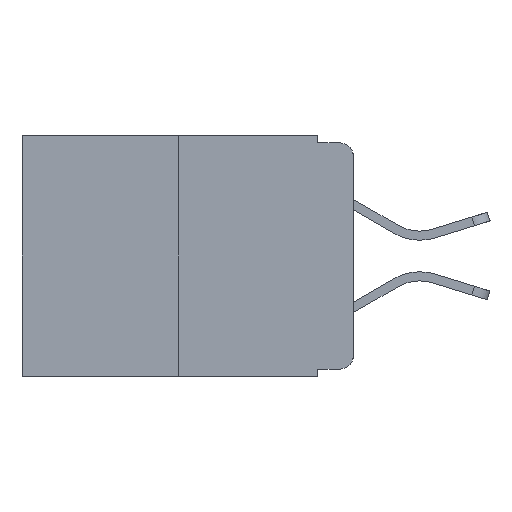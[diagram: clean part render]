
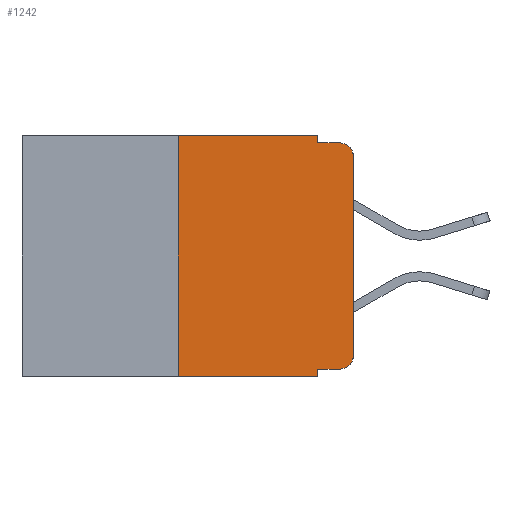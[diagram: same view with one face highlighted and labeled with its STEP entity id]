
A CAD part, left-side view. The second image highlights one B-rep face of the part: STEP entity #1242.
In plain terms, the highlighted planar face has unit normal (-1, 0, 0).
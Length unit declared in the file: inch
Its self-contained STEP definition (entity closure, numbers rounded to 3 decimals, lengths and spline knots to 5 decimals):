
#228 = DIRECTION ( 'NONE',  ( -1., 0., 0. ) ) ;
#306 = CARTESIAN_POINT ( 'NONE',  ( 0., 0.02, -0.333 ) ) ;
#309 = ORIENTED_EDGE ( 'NONE', *, *, #1476, .F. ) ;
#328 = DIRECTION ( 'NONE',  ( 0., 0., -1. ) ) ;
#923 = ORIENTED_EDGE ( 'NONE', *, *, #10424, .F. ) ;
#1242 = ADVANCED_FACE ( 'NONE', ( #10671 ), #13701, .F. ) ;
#1476 = EDGE_CURVE ( 'NONE', #9317, #11603, #1661, .T. ) ;
#1482 = VERTEX_POINT ( 'NONE', #10242 ) ;
#1661 = LINE ( 'NONE', #7023, #12177 ) ;
#1793 = LINE ( 'NONE', #8802, #4689 ) ;
#1803 = EDGE_LOOP ( 'NONE', ( #9860, #7399, #8414, #3017, #309, #9375, #8250, #923, #7599, #9241 ) ) ;
#2232 = VECTOR ( 'NONE', #11057, 39.37008 ) ;
#2859 = VERTEX_POINT ( 'NONE', #306 ) ;
#3017 = ORIENTED_EDGE ( 'NONE', *, *, #11734, .F. ) ;
#3085 = CARTESIAN_POINT ( 'NONE',  ( 0., 0.051, -0.01 ) ) ;
#3088 = VERTEX_POINT ( 'NONE', #3085 ) ;
#3152 = AXIS2_PLACEMENT_3D ( 'NONE', #6878, #228, #7946 ) ;
#3356 = VERTEX_POINT ( 'NONE', #5679 ) ;
#3462 = DIRECTION ( 'NONE',  ( 0., 0., -1. ) ) ;
#3478 = EDGE_CURVE ( 'NONE', #1482, #8459, #10699, .T. ) ;
#3678 = DIRECTION ( 'NONE',  ( 0., 0., 1. ) ) ;
#3749 = CARTESIAN_POINT ( 'NONE',  ( 0., 0., -0.313 ) ) ;
#3928 = LINE ( 'NONE', #10070, #9602 ) ;
#4041 = CARTESIAN_POINT ( 'NONE',  ( 0., 0.473, 0. ) ) ;
#4231 = LINE ( 'NONE', #12074, #12490 ) ;
#4430 = LINE ( 'NONE', #9846, #6610 ) ;
#4689 = VECTOR ( 'NONE', #12808, 39.37008 ) ;
#4858 = CARTESIAN_POINT ( 'NONE',  ( 0., 0.051, -0.01 ) ) ;
#4897 = DIRECTION ( 'NONE',  ( 0., 0., -1. ) ) ;
#5603 = CARTESIAN_POINT ( 'NONE',  ( 0., 0.02, -0.03 ) ) ;
#5679 = CARTESIAN_POINT ( 'NONE',  ( 0., 0.051, -0.333 ) ) ;
#5881 = CARTESIAN_POINT ( 'NONE',  ( 0., 0.051, -0.343 ) ) ;
#5893 = AXIS2_PLACEMENT_3D ( 'NONE', #5603, #12779, #6688 ) ;
#6195 = CARTESIAN_POINT ( 'NONE',  ( 0., 0.25, 0. ) ) ;
#6610 = VECTOR ( 'NONE', #3462, 39.37008 ) ;
#6688 = DIRECTION ( 'NONE',  ( 0., 0., -1. ) ) ;
#6878 = CARTESIAN_POINT ( 'NONE',  ( 0., 0.02, -0.313 ) ) ;
#6897 = LINE ( 'NONE', #4858, #7230 ) ;
#6948 = LINE ( 'NONE', #12994, #12060 ) ;
#7023 = CARTESIAN_POINT ( 'NONE',  ( 0., 0.473, 0. ) ) ;
#7049 = CIRCLE ( 'NONE', #5893, 0.02 ) ;
#7230 = VECTOR ( 'NONE', #13093, 39.37008 ) ;
#7399 = ORIENTED_EDGE ( 'NONE', *, *, #13064, .T. ) ;
#7599 = ORIENTED_EDGE ( 'NONE', *, *, #9749, .T. ) ;
#7946 = DIRECTION ( 'NONE',  ( 0., 0., -1. ) ) ;
#8250 = ORIENTED_EDGE ( 'NONE', *, *, #3478, .T. ) ;
#8260 = CARTESIAN_POINT ( 'NONE',  ( 0., 0.02, -0.01 ) ) ;
#8414 = ORIENTED_EDGE ( 'NONE', *, *, #12384, .F. ) ;
#8459 = VERTEX_POINT ( 'NONE', #5881 ) ;
#8802 = CARTESIAN_POINT ( 'NONE',  ( 0., 0., 0. ) ) ;
#9038 = EDGE_CURVE ( 'NONE', #2859, #12388, #11490, .T. ) ;
#9241 = ORIENTED_EDGE ( 'NONE', *, *, #9038, .T. ) ;
#9317 = VERTEX_POINT ( 'NONE', #6195 ) ;
#9375 = ORIENTED_EDGE ( 'NONE', *, *, #11083, .F. ) ;
#9602 = VECTOR ( 'NONE', #11071, 39.37008 ) ;
#9749 = EDGE_CURVE ( 'NONE', #3356, #2859, #3928, .T. ) ;
#9812 = DIRECTION ( 'NONE',  ( 0., -1., 0. ) ) ;
#9846 = CARTESIAN_POINT ( 'NONE',  ( 0., 0.051, 0. ) ) ;
#9860 = ORIENTED_EDGE ( 'NONE', *, *, #13747, .T. ) ;
#10070 = CARTESIAN_POINT ( 'NONE',  ( 0., 0.051, -0.333 ) ) ;
#10162 = DIRECTION ( 'NONE',  ( 1., 0., 0. ) ) ;
#10242 = CARTESIAN_POINT ( 'NONE',  ( 0., 0.25, -0.343 ) ) ;
#10372 = CARTESIAN_POINT ( 'NONE',  ( 0., 0., -0.03 ) ) ;
#10424 = EDGE_CURVE ( 'NONE', #3356, #8459, #4430, .T. ) ;
#10671 = FACE_OUTER_BOUND ( 'NONE', #1803, .T. ) ;
#10699 = LINE ( 'NONE', #11126, #2232 ) ;
#10763 = VERTEX_POINT ( 'NONE', #10372 ) ;
#11057 = DIRECTION ( 'NONE',  ( 0., -1., 0. ) ) ;
#11071 = DIRECTION ( 'NONE',  ( 0., -1., 0. ) ) ;
#11083 = EDGE_CURVE ( 'NONE', #1482, #9317, #6948, .T. ) ;
#11126 = CARTESIAN_POINT ( 'NONE',  ( 0., 0.473, -0.343 ) ) ;
#11490 = CIRCLE ( 'NONE', #3152, 0.02 ) ;
#11603 = VERTEX_POINT ( 'NONE', #12857 ) ;
#11734 = EDGE_CURVE ( 'NONE', #11603, #3088, #4231, .T. ) ;
#12060 = VECTOR ( 'NONE', #3678, 39.37008 ) ;
#12074 = CARTESIAN_POINT ( 'NONE',  ( 0., 0.051, 0. ) ) ;
#12177 = VECTOR ( 'NONE', #9812, 39.37008 ) ;
#12384 = EDGE_CURVE ( 'NONE', #3088, #12497, #6897, .T. ) ;
#12388 = VERTEX_POINT ( 'NONE', #3749 ) ;
#12490 = VECTOR ( 'NONE', #328, 39.37008 ) ;
#12497 = VERTEX_POINT ( 'NONE', #8260 ) ;
#12779 = DIRECTION ( 'NONE',  ( -1., 0., 0. ) ) ;
#12808 = DIRECTION ( 'NONE',  ( 0., 0., 1. ) ) ;
#12857 = CARTESIAN_POINT ( 'NONE',  ( 0., 0.051, 0. ) ) ;
#12994 = CARTESIAN_POINT ( 'NONE',  ( 0., 0.25, 0. ) ) ;
#13064 = EDGE_CURVE ( 'NONE', #10763, #12497, #7049, .T. ) ;
#13093 = DIRECTION ( 'NONE',  ( 0., -1., 0. ) ) ;
#13632 = AXIS2_PLACEMENT_3D ( 'NONE', #4041, #10162, #4897 ) ;
#13701 = PLANE ( 'NONE',  #13632 ) ;
#13747 = EDGE_CURVE ( 'NONE', #12388, #10763, #1793, .T. ) ;
